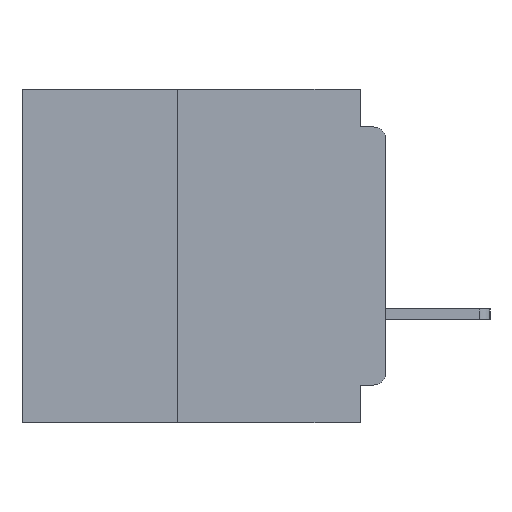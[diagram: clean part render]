
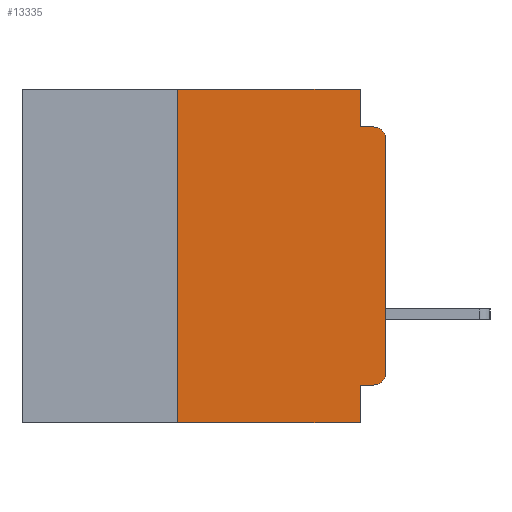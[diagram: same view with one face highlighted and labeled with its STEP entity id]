
A CAD part, left-side view. The second image highlights one B-rep face of the part: STEP entity #13335.
In plain terms, the highlighted planar face has unit normal (-1, 0, 0).
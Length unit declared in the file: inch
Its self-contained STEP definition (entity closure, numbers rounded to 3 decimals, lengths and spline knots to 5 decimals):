
#1153 = ORIENTED_EDGE ( 'NONE', *, *, #38669, .T. ) ;
#1305 = CARTESIAN_POINT ( 'NONE',  ( 0., 0.25, -0.4 ) ) ;
#1658 = CARTESIAN_POINT ( 'NONE',  ( 0., 0.437, 0. ) ) ;
#1934 = VECTOR ( 'NONE', #30577, 39.37008 ) ;
#2477 = VERTEX_POINT ( 'NONE', #12269 ) ;
#2793 = VERTEX_POINT ( 'NONE', #23285 ) ;
#3156 = FACE_OUTER_BOUND ( 'NONE', #7814, .T. ) ;
#3234 = ORIENTED_EDGE ( 'NONE', *, *, #35578, .F. ) ;
#4946 = DIRECTION ( 'NONE',  ( 0., 0., -1. ) ) ;
#4967 = ORIENTED_EDGE ( 'NONE', *, *, #5768, .F. ) ;
#5373 = CARTESIAN_POINT ( 'NONE',  ( 0., 0.031, -0.4 ) ) ;
#5405 = CARTESIAN_POINT ( 'NONE',  ( 0., 0.015, -0.06 ) ) ;
#5768 = EDGE_CURVE ( 'NONE', #2793, #6480, #9578, .T. ) ;
#6257 = CARTESIAN_POINT ( 'NONE',  ( 0., 0.437, -0.4 ) ) ;
#6480 = VERTEX_POINT ( 'NONE', #5373 ) ;
#7278 = VERTEX_POINT ( 'NONE', #25630 ) ;
#7660 = CIRCLE ( 'NONE', #26272, 0.015 ) ;
#7814 = EDGE_LOOP ( 'NONE', ( #28686, #12569, #31501, #24069, #3234, #27013, #1153, #4967, #14798, #11381 ) ) ;
#8106 = CARTESIAN_POINT ( 'NONE',  ( 0., 0.031, -0.4 ) ) ;
#8654 = DIRECTION ( 'NONE',  ( 0., 0., -1. ) ) ;
#8847 = LINE ( 'NONE', #41485, #33401 ) ;
#9068 = VERTEX_POINT ( 'NONE', #28260 ) ;
#9578 = LINE ( 'NONE', #8106, #1934 ) ;
#9849 = LINE ( 'NONE', #12816, #26977 ) ;
#10168 = EDGE_CURVE ( 'NONE', #22447, #37495, #33107, .T. ) ;
#11153 = CARTESIAN_POINT ( 'NONE',  ( 0., 0., -0.06 ) ) ;
#11326 = PLANE ( 'NONE',  #18130 ) ;
#11381 = ORIENTED_EDGE ( 'NONE', *, *, #13216, .T. ) ;
#11519 = VERTEX_POINT ( 'NONE', #11153 ) ;
#12269 = CARTESIAN_POINT ( 'NONE',  ( 0., 0.015, -0.045 ) ) ;
#12569 = ORIENTED_EDGE ( 'NONE', *, *, #35366, .T. ) ;
#12816 = CARTESIAN_POINT ( 'NONE',  ( 0., 0., -0.355 ) ) ;
#13216 = EDGE_CURVE ( 'NONE', #31410, #9068, #32833, .T. ) ;
#13335 = ADVANCED_FACE ( 'NONE', ( #3156 ), #11326, .F. ) ;
#14349 = VERTEX_POINT ( 'NONE', #1305 ) ;
#14798 = ORIENTED_EDGE ( 'NONE', *, *, #27214, .F. ) ;
#15143 = CARTESIAN_POINT ( 'NONE',  ( 0., 0.031, 0. ) ) ;
#15594 = CARTESIAN_POINT ( 'NONE',  ( 0., 0., -0.045 ) ) ;
#15952 = EDGE_CURVE ( 'NONE', #14349, #7278, #21069, .T. ) ;
#16069 = DIRECTION ( 'NONE',  ( 0., 0., 1. ) ) ;
#16752 = CARTESIAN_POINT ( 'NONE',  ( 0., 0.015, -0.355 ) ) ;
#17108 = CARTESIAN_POINT ( 'NONE',  ( 0., 0.015, -0.34 ) ) ;
#18130 = AXIS2_PLACEMENT_3D ( 'NONE', #1658, #24298, #4946 ) ;
#20356 = DIRECTION ( 'NONE',  ( 0., 0., -1. ) ) ;
#21069 = LINE ( 'NONE', #39960, #36981 ) ;
#21252 = LINE ( 'NONE', #15594, #28792 ) ;
#22447 = VERTEX_POINT ( 'NONE', #34519 ) ;
#23285 = CARTESIAN_POINT ( 'NONE',  ( 0., 0.031, -0.355 ) ) ;
#23296 = VECTOR ( 'NONE', #38250, 39.37008 ) ;
#23666 = EDGE_CURVE ( 'NONE', #37495, #2477, #21252, .T. ) ;
#24069 = ORIENTED_EDGE ( 'NONE', *, *, #10168, .F. ) ;
#24215 = DIRECTION ( 'NONE',  ( 0., 0., 1. ) ) ;
#24298 = DIRECTION ( 'NONE',  ( 1., 0., 0. ) ) ;
#25315 = DIRECTION ( 'NONE',  ( 0., -1., 0. ) ) ;
#25595 = DIRECTION ( 'NONE',  ( 0., -1., 0. ) ) ;
#25630 = CARTESIAN_POINT ( 'NONE',  ( 0., 0.25, 0. ) ) ;
#26272 = AXIS2_PLACEMENT_3D ( 'NONE', #5405, #27939, #8654 ) ;
#26977 = VECTOR ( 'NONE', #28816, 39.37008 ) ;
#27013 = ORIENTED_EDGE ( 'NONE', *, *, #15952, .F. ) ;
#27214 = EDGE_CURVE ( 'NONE', #31410, #2793, #9849, .T. ) ;
#27229 = EDGE_CURVE ( 'NONE', #9068, #11519, #8847, .T. ) ;
#27939 = DIRECTION ( 'NONE',  ( -1., 0., 0. ) ) ;
#28260 = CARTESIAN_POINT ( 'NONE',  ( 0., 0., -0.34 ) ) ;
#28686 = ORIENTED_EDGE ( 'NONE', *, *, #27229, .T. ) ;
#28792 = VECTOR ( 'NONE', #25315, 39.37008 ) ;
#28816 = DIRECTION ( 'NONE',  ( 0., 1., 0. ) ) ;
#29036 = CARTESIAN_POINT ( 'NONE',  ( 0., 0.437, 0. ) ) ;
#30577 = DIRECTION ( 'NONE',  ( 0., 0., -1. ) ) ;
#31094 = DIRECTION ( 'NONE',  ( 0., 0., -1. ) ) ;
#31410 = VERTEX_POINT ( 'NONE', #16752 ) ;
#31501 = ORIENTED_EDGE ( 'NONE', *, *, #23666, .F. ) ;
#31822 = AXIS2_PLACEMENT_3D ( 'NONE', #17108, #39373, #20356 ) ;
#32141 = VECTOR ( 'NONE', #31094, 39.37008 ) ;
#32740 = LINE ( 'NONE', #29036, #23296 ) ;
#32833 = CIRCLE ( 'NONE', #31822, 0.015 ) ;
#32941 = VECTOR ( 'NONE', #25595, 39.37008 ) ;
#33107 = LINE ( 'NONE', #15143, #32141 ) ;
#33401 = VECTOR ( 'NONE', #16069, 39.37008 ) ;
#33936 = LINE ( 'NONE', #6257, #32941 ) ;
#34519 = CARTESIAN_POINT ( 'NONE',  ( 0., 0.031, 0. ) ) ;
#35366 = EDGE_CURVE ( 'NONE', #11519, #2477, #7660, .T. ) ;
#35578 = EDGE_CURVE ( 'NONE', #7278, #22447, #32740, .T. ) ;
#36981 = VECTOR ( 'NONE', #24215, 39.37008 ) ;
#37142 = CARTESIAN_POINT ( 'NONE',  ( 0., 0.031, -0.045 ) ) ;
#37495 = VERTEX_POINT ( 'NONE', #37142 ) ;
#38250 = DIRECTION ( 'NONE',  ( 0., -1., 0. ) ) ;
#38669 = EDGE_CURVE ( 'NONE', #14349, #6480, #33936, .T. ) ;
#39373 = DIRECTION ( 'NONE',  ( -1., 0., 0. ) ) ;
#39960 = CARTESIAN_POINT ( 'NONE',  ( 0., 0.25, -0.4 ) ) ;
#41485 = CARTESIAN_POINT ( 'NONE',  ( 0., 0., 0. ) ) ;
